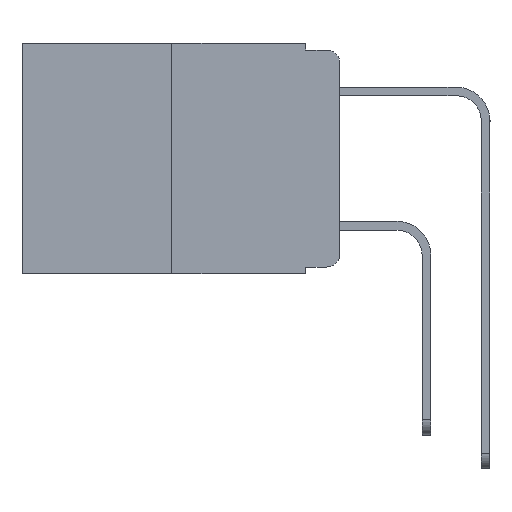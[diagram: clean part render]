
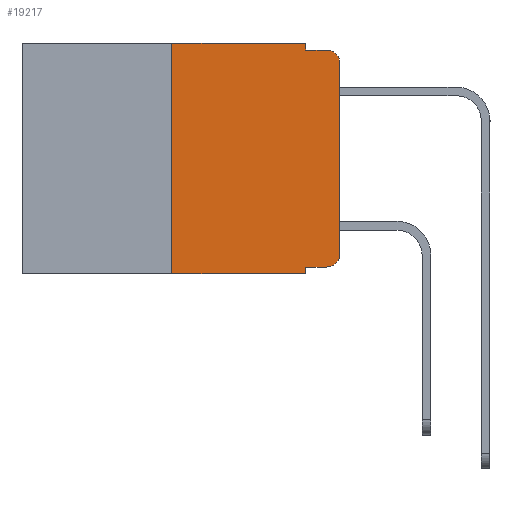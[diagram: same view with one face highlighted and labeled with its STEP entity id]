
A CAD part, left-side view. The second image highlights one B-rep face of the part: STEP entity #19217.
In plain terms, the highlighted planar face has unit normal (-1, 0, 0).
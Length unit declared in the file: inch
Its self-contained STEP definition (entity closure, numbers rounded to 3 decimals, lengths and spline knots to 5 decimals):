
#154 = EDGE_LOOP ( 'NONE', ( #13872, #5760, #19647, #9042, #1832, #7154, #12294, #22570, #19110, #8525 ) ) ;
#265 = CIRCLE ( 'NONE', #12039, 0.02 ) ;
#326 = CARTESIAN_POINT ( 'NONE',  ( 0., 0.25, -0.343 ) ) ;
#420 = VERTEX_POINT ( 'NONE', #3280 ) ;
#505 = VECTOR ( 'NONE', #12864, 39.37008 ) ;
#648 = DIRECTION ( 'NONE',  ( 0., -1., 0. ) ) ;
#1353 = CARTESIAN_POINT ( 'NONE',  ( 0., 0., -0.03 ) ) ;
#1549 = CARTESIAN_POINT ( 'NONE',  ( 0., 0.02, -0.03 ) ) ;
#1817 = EDGE_CURVE ( 'NONE', #19700, #8839, #6791, .T. ) ;
#1832 = ORIENTED_EDGE ( 'NONE', *, *, #7411, .F. ) ;
#2021 = VECTOR ( 'NONE', #17535, 39.37008 ) ;
#2425 = VERTEX_POINT ( 'NONE', #4943 ) ;
#2441 = CARTESIAN_POINT ( 'NONE',  ( 0., 0.473, -0.343 ) ) ;
#2631 = DIRECTION ( 'NONE',  ( 1., 0., 0. ) ) ;
#2996 = CARTESIAN_POINT ( 'NONE',  ( 0., 0.02, -0.333 ) ) ;
#3020 = CARTESIAN_POINT ( 'NONE',  ( 0., 0.25, 0. ) ) ;
#3022 = VERTEX_POINT ( 'NONE', #21590 ) ;
#3056 = EDGE_CURVE ( 'NONE', #14055, #3238, #10533, .T. ) ;
#3138 = CIRCLE ( 'NONE', #14592, 0.02 ) ;
#3237 = VECTOR ( 'NONE', #648, 39.37008 ) ;
#3238 = VERTEX_POINT ( 'NONE', #9625 ) ;
#3280 = CARTESIAN_POINT ( 'NONE',  ( 0., 0.051, -0.333 ) ) ;
#3403 = DIRECTION ( 'NONE',  ( 0., 0., -1. ) ) ;
#4504 = CARTESIAN_POINT ( 'NONE',  ( 0., 0.051, 0. ) ) ;
#4943 = CARTESIAN_POINT ( 'NONE',  ( 0., 0., -0.313 ) ) ;
#5473 = EDGE_CURVE ( 'NONE', #3238, #3022, #11533, .T. ) ;
#5640 = EDGE_CURVE ( 'NONE', #19700, #7209, #7934, .T. ) ;
#5760 = ORIENTED_EDGE ( 'NONE', *, *, #7798, .T. ) ;
#6038 = CARTESIAN_POINT ( 'NONE',  ( 0., 0.02, -0.313 ) ) ;
#6282 = DIRECTION ( 'NONE',  ( 0., 0., 1. ) ) ;
#6455 = VERTEX_POINT ( 'NONE', #1353 ) ;
#6791 = LINE ( 'NONE', #3020, #2021 ) ;
#6928 = VECTOR ( 'NONE', #10760, 39.37008 ) ;
#7154 = ORIENTED_EDGE ( 'NONE', *, *, #1817, .F. ) ;
#7209 = VERTEX_POINT ( 'NONE', #10630 ) ;
#7411 = EDGE_CURVE ( 'NONE', #8839, #14055, #8707, .T. ) ;
#7779 = DIRECTION ( 'NONE',  ( 0., 0., -1. ) ) ;
#7798 = EDGE_CURVE ( 'NONE', #6455, #3022, #265, .T. ) ;
#7934 = LINE ( 'NONE', #2441, #3237 ) ;
#8163 = DIRECTION ( 'NONE',  ( 0., -1., 0. ) ) ;
#8525 = ORIENTED_EDGE ( 'NONE', *, *, #16308, .T. ) ;
#8707 = LINE ( 'NONE', #19738, #17914 ) ;
#8717 = VECTOR ( 'NONE', #13142, 39.37008 ) ;
#8839 = VERTEX_POINT ( 'NONE', #21036 ) ;
#9042 = ORIENTED_EDGE ( 'NONE', *, *, #3056, .F. ) ;
#9625 = CARTESIAN_POINT ( 'NONE',  ( 0., 0.051, -0.01 ) ) ;
#9633 = LINE ( 'NONE', #18419, #14221 ) ;
#9647 = CARTESIAN_POINT ( 'NONE',  ( 0., 0.473, 0. ) ) ;
#10128 = VECTOR ( 'NONE', #8163, 39.37008 ) ;
#10420 = EDGE_CURVE ( 'NONE', #2425, #6455, #9633, .T. ) ;
#10533 = LINE ( 'NONE', #18209, #505 ) ;
#10630 = CARTESIAN_POINT ( 'NONE',  ( 0., 0.051, -0.343 ) ) ;
#10760 = DIRECTION ( 'NONE',  ( 0., -1., 0. ) ) ;
#11075 = DIRECTION ( 'NONE',  ( 0., -1., 0. ) ) ;
#11533 = LINE ( 'NONE', #12498, #6928 ) ;
#12039 = AXIS2_PLACEMENT_3D ( 'NONE', #1549, #13840, #3403 ) ;
#12294 = ORIENTED_EDGE ( 'NONE', *, *, #5640, .T. ) ;
#12498 = CARTESIAN_POINT ( 'NONE',  ( 0., 0.051, -0.01 ) ) ;
#12645 = AXIS2_PLACEMENT_3D ( 'NONE', #9647, #2631, #14836 ) ;
#12864 = DIRECTION ( 'NONE',  ( 0., 0., -1. ) ) ;
#12869 = CARTESIAN_POINT ( 'NONE',  ( 0., 0.051, 0. ) ) ;
#13116 = PLANE ( 'NONE',  #12645 ) ;
#13142 = DIRECTION ( 'NONE',  ( 0., 0., -1. ) ) ;
#13840 = DIRECTION ( 'NONE',  ( -1., 0., 0. ) ) ;
#13872 = ORIENTED_EDGE ( 'NONE', *, *, #10420, .T. ) ;
#14055 = VERTEX_POINT ( 'NONE', #12869 ) ;
#14221 = VECTOR ( 'NONE', #6282, 39.37008 ) ;
#14592 = AXIS2_PLACEMENT_3D ( 'NONE', #6038, #18169, #7779 ) ;
#14836 = DIRECTION ( 'NONE',  ( 0., 0., -1. ) ) ;
#15884 = VERTEX_POINT ( 'NONE', #2996 ) ;
#16308 = EDGE_CURVE ( 'NONE', #15884, #2425, #3138, .T. ) ;
#16758 = CARTESIAN_POINT ( 'NONE',  ( 0., 0.051, -0.333 ) ) ;
#17535 = DIRECTION ( 'NONE',  ( 0., 0., 1. ) ) ;
#17914 = VECTOR ( 'NONE', #11075, 39.37008 ) ;
#18169 = DIRECTION ( 'NONE',  ( -1., 0., 0. ) ) ;
#18209 = CARTESIAN_POINT ( 'NONE',  ( 0., 0.051, 0. ) ) ;
#18419 = CARTESIAN_POINT ( 'NONE',  ( 0., 0., 0. ) ) ;
#18708 = EDGE_CURVE ( 'NONE', #420, #15884, #18827, .T. ) ;
#18827 = LINE ( 'NONE', #16758, #10128 ) ;
#19110 = ORIENTED_EDGE ( 'NONE', *, *, #18708, .T. ) ;
#19217 = ADVANCED_FACE ( 'NONE', ( #21735 ), #13116, .F. ) ;
#19647 = ORIENTED_EDGE ( 'NONE', *, *, #5473, .F. ) ;
#19700 = VERTEX_POINT ( 'NONE', #326 ) ;
#19738 = CARTESIAN_POINT ( 'NONE',  ( 0., 0.473, 0. ) ) ;
#19879 = EDGE_CURVE ( 'NONE', #420, #7209, #22501, .T. ) ;
#21036 = CARTESIAN_POINT ( 'NONE',  ( 0., 0.25, 0. ) ) ;
#21590 = CARTESIAN_POINT ( 'NONE',  ( 0., 0.02, -0.01 ) ) ;
#21735 = FACE_OUTER_BOUND ( 'NONE', #154, .T. ) ;
#22501 = LINE ( 'NONE', #4504, #8717 ) ;
#22570 = ORIENTED_EDGE ( 'NONE', *, *, #19879, .F. ) ;
